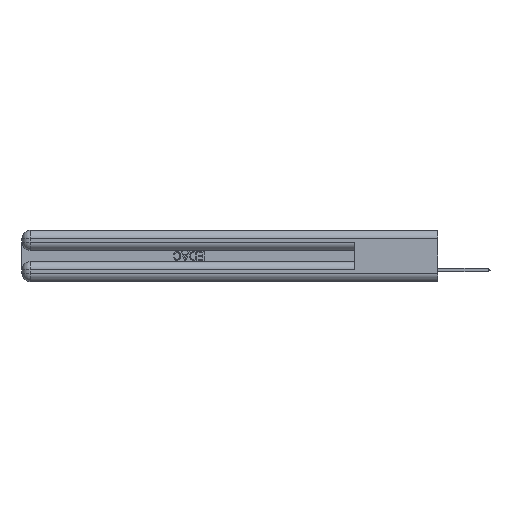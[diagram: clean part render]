
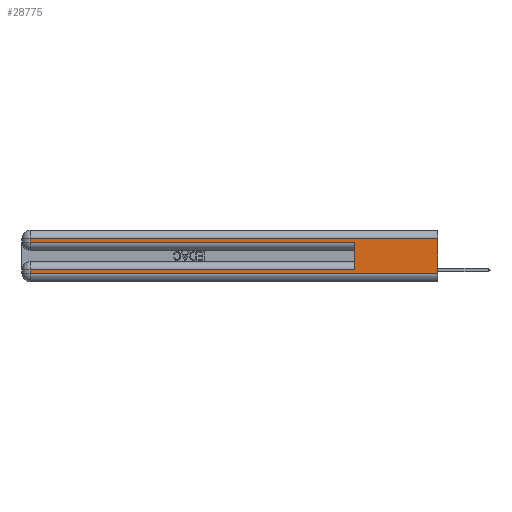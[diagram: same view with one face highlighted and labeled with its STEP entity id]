
A CAD part, left-side view. The second image highlights one B-rep face of the part: STEP entity #28775.
In plain terms, the highlighted planar face has unit normal (-1, 0, 0).
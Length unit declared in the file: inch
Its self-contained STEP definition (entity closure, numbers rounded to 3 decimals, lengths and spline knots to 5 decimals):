
#423 = CARTESIAN_POINT ( 'NONE',  ( 0., 0., 0.06 ) ) ;
#802 = DIRECTION ( 'NONE',  ( 0., 0., -1. ) ) ;
#835 = DIRECTION ( 'NONE',  ( 0., -1., 0. ) ) ;
#1069 = CARTESIAN_POINT ( 'NONE',  ( 0., 0., 0.37 ) ) ;
#1692 = CARTESIAN_POINT ( 'NONE',  ( 0., 2.94, 0.06 ) ) ;
#2290 = DIRECTION ( 'NONE',  ( 0., -1., 0. ) ) ;
#2451 = CARTESIAN_POINT ( 'NONE',  ( 0., 0., 0.06 ) ) ;
#3302 = VERTEX_POINT ( 'NONE', #27765 ) ;
#4435 = LINE ( 'NONE', #39110, #28693 ) ;
#4473 = DIRECTION ( 'NONE',  ( 0., 1., 0. ) ) ;
#5582 = ORIENTED_EDGE ( 'NONE', *, *, #18818, .T. ) ;
#6936 = VERTEX_POINT ( 'NONE', #2451 ) ;
#7564 = EDGE_LOOP ( 'NONE', ( #29983, #32917, #29606, #5582, #16462, #24221, #36277, #18516 ) ) ;
#7642 = CARTESIAN_POINT ( 'NONE',  ( 0., 0.6, 0.145 ) ) ;
#8225 = EDGE_CURVE ( 'NONE', #8566, #3302, #19900, .T. ) ;
#8462 = DIRECTION ( 'NONE',  ( 0., 0., -1. ) ) ;
#8566 = VERTEX_POINT ( 'NONE', #11337 ) ;
#8605 = LINE ( 'NONE', #7642, #25777 ) ;
#8660 = VERTEX_POINT ( 'NONE', #20421 ) ;
#10259 = LINE ( 'NONE', #423, #29801 ) ;
#10313 = EDGE_CURVE ( 'NONE', #38413, #12809, #19236, .T. ) ;
#11056 = EDGE_CURVE ( 'NONE', #3302, #14806, #4435, .T. ) ;
#11337 = CARTESIAN_POINT ( 'NONE',  ( 0., 0., 0.31 ) ) ;
#11889 = DIRECTION ( 'NONE',  ( 0., 0., -1. ) ) ;
#11966 = EDGE_CURVE ( 'NONE', #24668, #8660, #8605, .T. ) ;
#12085 = AXIS2_PLACEMENT_3D ( 'NONE', #15383, #32560, #16777 ) ;
#12637 = VECTOR ( 'NONE', #2290, 39.37008 ) ;
#12809 = VERTEX_POINT ( 'NONE', #1692 ) ;
#13451 = EDGE_CURVE ( 'NONE', #8566, #6936, #24541, .T. ) ;
#14806 = VERTEX_POINT ( 'NONE', #23901 ) ;
#15383 = CARTESIAN_POINT ( 'NONE',  ( 0., 0., 0.37 ) ) ;
#16450 = VECTOR ( 'NONE', #802, 39.37008 ) ;
#16462 = ORIENTED_EDGE ( 'NONE', *, *, #11966, .F. ) ;
#16777 = DIRECTION ( 'NONE',  ( 0., 0., -1. ) ) ;
#18516 = ORIENTED_EDGE ( 'NONE', *, *, #20873, .T. ) ;
#18729 = DIRECTION ( 'NONE',  ( 0., 1., 0. ) ) ;
#18818 = EDGE_CURVE ( 'NONE', #14806, #8660, #39259, .T. ) ;
#19236 = LINE ( 'NONE', #35742, #33477 ) ;
#19900 = LINE ( 'NONE', #39159, #26078 ) ;
#20421 = CARTESIAN_POINT ( 'NONE',  ( 0., 0.6, 0.285 ) ) ;
#20873 = EDGE_CURVE ( 'NONE', #12809, #6936, #10259, .T. ) ;
#23882 = VECTOR ( 'NONE', #4473, 39.37008 ) ;
#23901 = CARTESIAN_POINT ( 'NONE',  ( 0., 2.94, 0.285 ) ) ;
#24062 = EDGE_CURVE ( 'NONE', #24668, #38413, #38532, .T. ) ;
#24221 = ORIENTED_EDGE ( 'NONE', *, *, #24062, .T. ) ;
#24541 = LINE ( 'NONE', #1069, #16450 ) ;
#24668 = VERTEX_POINT ( 'NONE', #35342 ) ;
#24848 = PLANE ( 'NONE',  #12085 ) ;
#25777 = VECTOR ( 'NONE', #27194, 39.37008 ) ;
#26078 = VECTOR ( 'NONE', #18729, 39.37008 ) ;
#27194 = DIRECTION ( 'NONE',  ( 0., 0., 1. ) ) ;
#27566 = CARTESIAN_POINT ( 'NONE',  ( 0., 0., 0.285 ) ) ;
#27765 = CARTESIAN_POINT ( 'NONE',  ( 0., 2.94, 0.31 ) ) ;
#27869 = CARTESIAN_POINT ( 'NONE',  ( 0., 2.94, 0.085 ) ) ;
#28397 = CARTESIAN_POINT ( 'NONE',  ( 0., 0., 0.085 ) ) ;
#28693 = VECTOR ( 'NONE', #11889, 39.37008 ) ;
#28775 = ADVANCED_FACE ( 'NONE', ( #29251 ), #24848, .F. ) ;
#29251 = FACE_OUTER_BOUND ( 'NONE', #7564, .T. ) ;
#29606 = ORIENTED_EDGE ( 'NONE', *, *, #11056, .T. ) ;
#29801 = VECTOR ( 'NONE', #835, 39.37008 ) ;
#29983 = ORIENTED_EDGE ( 'NONE', *, *, #13451, .F. ) ;
#32560 = DIRECTION ( 'NONE',  ( 1., 0., 0. ) ) ;
#32917 = ORIENTED_EDGE ( 'NONE', *, *, #8225, .T. ) ;
#33477 = VECTOR ( 'NONE', #8462, 39.37008 ) ;
#35342 = CARTESIAN_POINT ( 'NONE',  ( 0., 0.6, 0.085 ) ) ;
#35742 = CARTESIAN_POINT ( 'NONE',  ( 0., 2.94, 0.37 ) ) ;
#36277 = ORIENTED_EDGE ( 'NONE', *, *, #10313, .T. ) ;
#38413 = VERTEX_POINT ( 'NONE', #27869 ) ;
#38532 = LINE ( 'NONE', #28397, #23882 ) ;
#39110 = CARTESIAN_POINT ( 'NONE',  ( 0., 2.94, 0.37 ) ) ;
#39159 = CARTESIAN_POINT ( 'NONE',  ( 0., 0., 0.31 ) ) ;
#39259 = LINE ( 'NONE', #27566, #12637 ) ;
